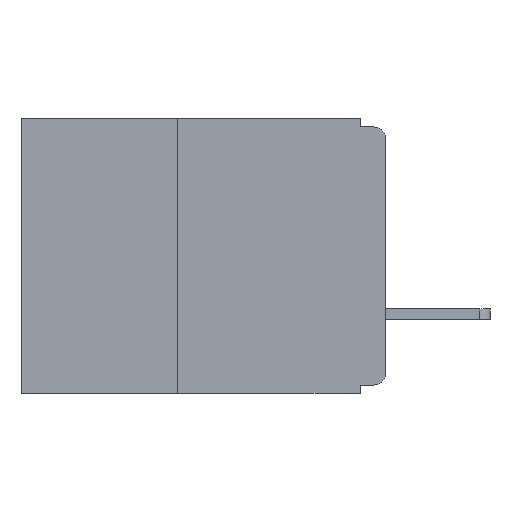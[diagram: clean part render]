
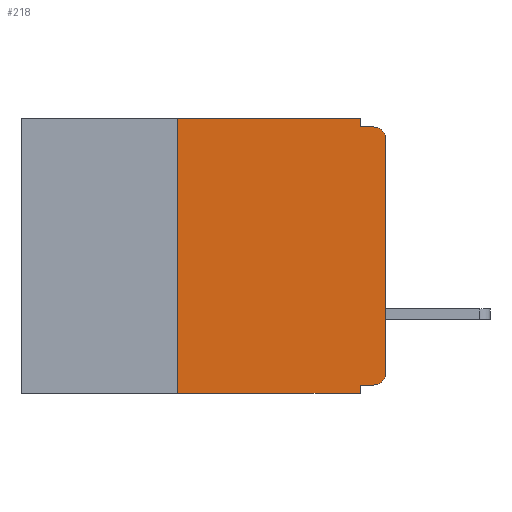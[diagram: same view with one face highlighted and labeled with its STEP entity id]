
A CAD part, left-side view. The second image highlights one B-rep face of the part: STEP entity #218.
In plain terms, the highlighted planar face has unit normal (-1, 0, 0).
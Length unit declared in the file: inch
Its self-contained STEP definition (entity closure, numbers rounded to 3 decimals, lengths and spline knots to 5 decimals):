
#218 = ADVANCED_FACE ( 'NONE', ( #18002 ), #5824, .F. ) ;
#979 = DIRECTION ( 'NONE',  ( 0., 0., -1. ) ) ;
#1158 = AXIS2_PLACEMENT_3D ( 'NONE', #23040, #10310, #25136 ) ;
#1681 = ORIENTED_EDGE ( 'NONE', *, *, #8383, .T. ) ;
#1803 = VECTOR ( 'NONE', #16913, 39.37008 ) ;
#2461 = LINE ( 'NONE', #4098, #1803 ) ;
#3822 = ORIENTED_EDGE ( 'NONE', *, *, #19208, .T. ) ;
#3936 = CARTESIAN_POINT ( 'NONE',  ( 0., 0.031, -0.01 ) ) ;
#4098 = CARTESIAN_POINT ( 'NONE',  ( 0., 0., -0.32 ) ) ;
#4406 = ORIENTED_EDGE ( 'NONE', *, *, #15776, .T. ) ;
#4531 = VECTOR ( 'NONE', #18290, 39.37008 ) ;
#4621 = LINE ( 'NONE', #13326, #15350 ) ;
#4940 = DIRECTION ( 'NONE',  ( 0., 0., -1. ) ) ;
#5816 = DIRECTION ( 'NONE',  ( 1., 0., 0. ) ) ;
#5824 = PLANE ( 'NONE',  #9614 ) ;
#6072 = CARTESIAN_POINT ( 'NONE',  ( 0., 0.015, -0.32 ) ) ;
#6810 = ORIENTED_EDGE ( 'NONE', *, *, #12084, .F. ) ;
#6852 = VERTEX_POINT ( 'NONE', #23891 ) ;
#7325 = DIRECTION ( 'NONE',  ( 0., -1., 0. ) ) ;
#7822 = CARTESIAN_POINT ( 'NONE',  ( 0., 0., -0.01 ) ) ;
#7960 = CARTESIAN_POINT ( 'NONE',  ( 0., 0.25, 0. ) ) ;
#8383 = EDGE_CURVE ( 'NONE', #11741, #12714, #15917, .T. ) ;
#8589 = VECTOR ( 'NONE', #27095, 39.37008 ) ;
#9123 = DIRECTION ( 'NONE',  ( -1., 0., 0. ) ) ;
#9164 = VERTEX_POINT ( 'NONE', #3936 ) ;
#9324 = EDGE_CURVE ( 'NONE', #6852, #9164, #4621, .T. ) ;
#9429 = DIRECTION ( 'NONE',  ( 0., 0., -1. ) ) ;
#9597 = VERTEX_POINT ( 'NONE', #16080 ) ;
#9614 = AXIS2_PLACEMENT_3D ( 'NONE', #26787, #5816, #9429 ) ;
#9931 = VECTOR ( 'NONE', #9970, 39.37008 ) ;
#9970 = DIRECTION ( 'NONE',  ( 0., -1., 0. ) ) ;
#10102 = DIRECTION ( 'NONE',  ( 0., -1., 0. ) ) ;
#10171 = CARTESIAN_POINT ( 'NONE',  ( 0., 0.25, -0.33 ) ) ;
#10310 = DIRECTION ( 'NONE',  ( -1., 0., 0. ) ) ;
#10521 = VECTOR ( 'NONE', #7325, 39.37008 ) ;
#10613 = LINE ( 'NONE', #7822, #9931 ) ;
#10709 = EDGE_CURVE ( 'NONE', #12714, #23414, #13286, .T. ) ;
#11152 = EDGE_LOOP ( 'NONE', ( #1681, #21494, #15535, #27383, #6810, #13872, #3822, #12243, #16898, #4406 ) ) ;
#11697 = CARTESIAN_POINT ( 'NONE',  ( 0., 0.031, -0.33 ) ) ;
#11741 = VERTEX_POINT ( 'NONE', #21170 ) ;
#12054 = CARTESIAN_POINT ( 'NONE',  ( 0., 0., -0.025 ) ) ;
#12084 = EDGE_CURVE ( 'NONE', #15726, #6852, #21822, .T. ) ;
#12243 = ORIENTED_EDGE ( 'NONE', *, *, #24004, .F. ) ;
#12281 = CARTESIAN_POINT ( 'NONE',  ( 0., 0.437, -0.33 ) ) ;
#12479 = VERTEX_POINT ( 'NONE', #17512 ) ;
#12714 = VERTEX_POINT ( 'NONE', #12054 ) ;
#13052 = CIRCLE ( 'NONE', #1158, 0.015 ) ;
#13116 = CARTESIAN_POINT ( 'NONE',  ( 0., 0.015, -0.01 ) ) ;
#13286 = CIRCLE ( 'NONE', #17936, 0.015 ) ;
#13326 = CARTESIAN_POINT ( 'NONE',  ( 0., 0.031, 0. ) ) ;
#13491 = VERTEX_POINT ( 'NONE', #6072 ) ;
#13715 = CARTESIAN_POINT ( 'NONE',  ( 0., 0.437, 0. ) ) ;
#13872 = ORIENTED_EDGE ( 'NONE', *, *, #26550, .F. ) ;
#14005 = CARTESIAN_POINT ( 'NONE',  ( 0., 0., 0. ) ) ;
#14525 = CARTESIAN_POINT ( 'NONE',  ( 0., 0.031, -0.32 ) ) ;
#15350 = VECTOR ( 'NONE', #4940, 39.37008 ) ;
#15535 = ORIENTED_EDGE ( 'NONE', *, *, #26487, .F. ) ;
#15726 = VERTEX_POINT ( 'NONE', #7960 ) ;
#15776 = EDGE_CURVE ( 'NONE', #13491, #11741, #13052, .T. ) ;
#15917 = LINE ( 'NONE', #14005, #4531 ) ;
#16080 = CARTESIAN_POINT ( 'NONE',  ( 0., 0.031, -0.33 ) ) ;
#16435 = LINE ( 'NONE', #11697, #21411 ) ;
#16898 = ORIENTED_EDGE ( 'NONE', *, *, #27456, .F. ) ;
#16913 = DIRECTION ( 'NONE',  ( 0., 1., 0. ) ) ;
#17512 = CARTESIAN_POINT ( 'NONE',  ( 0., 0.25, -0.33 ) ) ;
#17555 = VERTEX_POINT ( 'NONE', #14525 ) ;
#17936 = AXIS2_PLACEMENT_3D ( 'NONE', #21868, #9123, #23968 ) ;
#18002 = FACE_OUTER_BOUND ( 'NONE', #11152, .T. ) ;
#18290 = DIRECTION ( 'NONE',  ( 0., 0., 1. ) ) ;
#19208 = EDGE_CURVE ( 'NONE', #12479, #9597, #26054, .T. ) ;
#20485 = VECTOR ( 'NONE', #10102, 39.37008 ) ;
#21170 = CARTESIAN_POINT ( 'NONE',  ( 0., 0., -0.305 ) ) ;
#21411 = VECTOR ( 'NONE', #979, 39.37008 ) ;
#21494 = ORIENTED_EDGE ( 'NONE', *, *, #10709, .T. ) ;
#21822 = LINE ( 'NONE', #13715, #10521 ) ;
#21868 = CARTESIAN_POINT ( 'NONE',  ( 0., 0.015, -0.025 ) ) ;
#23040 = CARTESIAN_POINT ( 'NONE',  ( 0., 0.015, -0.305 ) ) ;
#23414 = VERTEX_POINT ( 'NONE', #13116 ) ;
#23891 = CARTESIAN_POINT ( 'NONE',  ( 0., 0.031, 0. ) ) ;
#23968 = DIRECTION ( 'NONE',  ( 0., 0., -1. ) ) ;
#24004 = EDGE_CURVE ( 'NONE', #17555, #9597, #16435, .T. ) ;
#25136 = DIRECTION ( 'NONE',  ( 0., 0., -1. ) ) ;
#25496 = LINE ( 'NONE', #10171, #8589 ) ;
#26054 = LINE ( 'NONE', #12281, #20485 ) ;
#26487 = EDGE_CURVE ( 'NONE', #9164, #23414, #10613, .T. ) ;
#26550 = EDGE_CURVE ( 'NONE', #12479, #15726, #25496, .T. ) ;
#26787 = CARTESIAN_POINT ( 'NONE',  ( 0., 0.437, 0. ) ) ;
#27095 = DIRECTION ( 'NONE',  ( 0., 0., 1. ) ) ;
#27383 = ORIENTED_EDGE ( 'NONE', *, *, #9324, .F. ) ;
#27456 = EDGE_CURVE ( 'NONE', #13491, #17555, #2461, .T. ) ;
